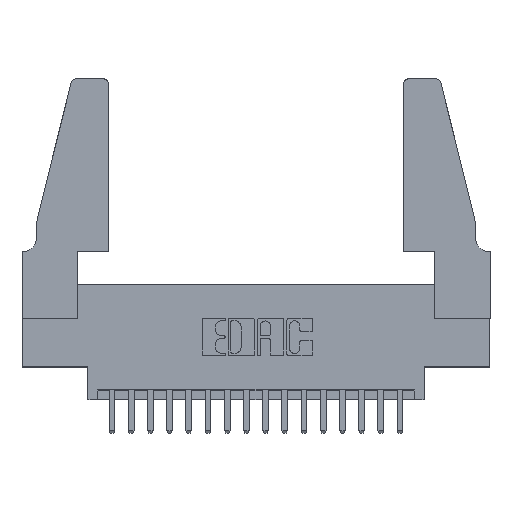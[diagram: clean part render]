
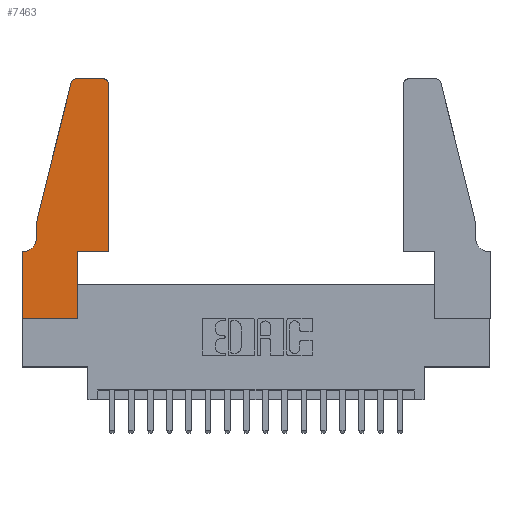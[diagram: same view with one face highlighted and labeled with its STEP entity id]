
A CAD part, top view. The second image highlights one B-rep face of the part: STEP entity #7463.
In plain terms, the highlighted planar face has unit normal (0, 0, 1).
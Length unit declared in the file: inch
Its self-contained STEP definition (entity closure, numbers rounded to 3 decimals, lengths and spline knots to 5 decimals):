
#109 = CARTESIAN_POINT ( 'NONE',  ( 0.0055, 0.35, 0.37 ) ) ;
#474 = ORIENTED_EDGE ( 'NONE', *, *, #11904, .T. ) ;
#642 = ORIENTED_EDGE ( 'NONE', *, *, #15482, .T. ) ;
#765 = DIRECTION ( 'NONE',  ( 0., 0., -1. ) ) ;
#843 = DIRECTION ( 'NONE',  ( -0.239, -0.971, 0. ) ) ;
#953 = LINE ( 'NONE', #1399, #3434 ) ;
#1150 = EDGE_CURVE ( 'NONE', #9525, #9662, #5143, .T. ) ;
#1267 = DIRECTION ( 'NONE',  ( 0., 1., 0. ) ) ;
#1284 = EDGE_CURVE ( 'NONE', #12994, #13766, #10468, .T. ) ;
#1294 = VECTOR ( 'NONE', #9110, 39.37008 ) ;
#1304 = CARTESIAN_POINT ( 'NONE',  ( 0.2605, 1.25, 0.37 ) ) ;
#1356 = ORIENTED_EDGE ( 'NONE', *, *, #17627, .T. ) ;
#1365 = LINE ( 'NONE', #4726, #8556 ) ;
#1399 = CARTESIAN_POINT ( 'NONE',  ( 0.4505, 0.35, 0.37 ) ) ;
#1490 = EDGE_CURVE ( 'NONE', #9662, #12390, #17792, .T. ) ;
#1530 = AXIS2_PLACEMENT_3D ( 'NONE', #3907, #13874, #5355 ) ;
#1618 = CARTESIAN_POINT ( 'NONE',  ( 0.0755, 0.5, 0.37 ) ) ;
#1721 = ORIENTED_EDGE ( 'NONE', *, *, #9318, .T. ) ;
#1859 = CARTESIAN_POINT ( 'NONE',  ( 0.2865, 0.35, 0.37 ) ) ;
#1992 = CARTESIAN_POINT ( 'NONE',  ( 0., 0., 0.37 ) ) ;
#2109 = DIRECTION ( 'NONE',  ( 1., 0., 0. ) ) ;
#2686 = CIRCLE ( 'NONE', #1530, 0.03 ) ;
#2865 = VECTOR ( 'NONE', #843, 39.37008 ) ;
#2963 = CARTESIAN_POINT ( 'NONE',  ( 0., 0.35, 0.37 ) ) ;
#3119 = AXIS2_PLACEMENT_3D ( 'NONE', #9359, #765, #10773 ) ;
#3434 = VECTOR ( 'NONE', #5691, 39.37008 ) ;
#3634 = EDGE_CURVE ( 'NONE', #13766, #15212, #13282, .T. ) ;
#3751 = LINE ( 'NONE', #10677, #18422 ) ;
#3825 = CARTESIAN_POINT ( 'NONE',  ( 0.2865, 0.35, 0.37 ) ) ;
#3907 = CARTESIAN_POINT ( 'NONE',  ( 0.284, 1.22, 0.37 ) ) ;
#3990 = LINE ( 'NONE', #1992, #6900 ) ;
#4007 = CARTESIAN_POINT ( 'NONE',  ( 0.0755, 0.42, 0.37 ) ) ;
#4099 = VERTEX_POINT ( 'NONE', #109 ) ;
#4253 = CARTESIAN_POINT ( 'NONE',  ( 0.4505, 1.22, 0.37 ) ) ;
#4267 = CARTESIAN_POINT ( 'NONE',  ( 0.284, 1.25, 0.37 ) ) ;
#4495 = DIRECTION ( 'NONE',  ( 1., 0., 0. ) ) ;
#4726 = CARTESIAN_POINT ( 'NONE',  ( 0.0755, 0.35, 0.37 ) ) ;
#5143 = LINE ( 'NONE', #15594, #1294 ) ;
#5355 = DIRECTION ( 'NONE',  ( 1., 0., 0. ) ) ;
#5691 = DIRECTION ( 'NONE',  ( 0., 1., 0. ) ) ;
#5715 = VECTOR ( 'NONE', #17340, 39.37008 ) ;
#5941 = CARTESIAN_POINT ( 'NONE',  ( 0.4205, 1.25, 0.37 ) ) ;
#5957 = EDGE_CURVE ( 'NONE', #12606, #12994, #2686, .T. ) ;
#6255 = DIRECTION ( 'NONE',  ( 0., 0., 1. ) ) ;
#6426 = EDGE_CURVE ( 'NONE', #12390, #6886, #3751, .T. ) ;
#6432 = CIRCLE ( 'NONE', #17276, 0.03 ) ;
#6886 = VERTEX_POINT ( 'NONE', #16083 ) ;
#6900 = VECTOR ( 'NONE', #14789, 39.37008 ) ;
#6916 = LINE ( 'NONE', #1304, #10248 ) ;
#7120 = EDGE_LOOP ( 'NONE', ( #474, #17174, #14389, #16852, #10218, #1721, #18307, #7163, #14049, #15892, #1356, #642 ) ) ;
#7163 = ORIENTED_EDGE ( 'NONE', *, *, #1150, .T. ) ;
#7463 = ADVANCED_FACE ( 'NONE', ( #16615 ), #10159, .T. ) ;
#8556 = VECTOR ( 'NONE', #9029, 39.37008 ) ;
#8744 = AXIS2_PLACEMENT_3D ( 'NONE', #2963, #13028, #4495 ) ;
#8820 = EDGE_CURVE ( 'NONE', #15212, #4099, #13684, .T. ) ;
#9029 = DIRECTION ( 'NONE',  ( -1., 0., 0. ) ) ;
#9110 = DIRECTION ( 'NONE',  ( 1., 0., 0. ) ) ;
#9318 = EDGE_CURVE ( 'NONE', #4099, #18301, #1365, .T. ) ;
#9359 = CARTESIAN_POINT ( 'NONE',  ( 0.0055, 0.42, 0.37 ) ) ;
#9525 = VERTEX_POINT ( 'NONE', #16526 ) ;
#9662 = VERTEX_POINT ( 'NONE', #15407 ) ;
#9889 = DIRECTION ( 'NONE',  ( -1., 0., 0. ) ) ;
#10159 = PLANE ( 'NONE',  #8744 ) ;
#10218 = ORIENTED_EDGE ( 'NONE', *, *, #8820, .T. ) ;
#10248 = VECTOR ( 'NONE', #9889, 39.37008 ) ;
#10468 = LINE ( 'NONE', #1618, #2865 ) ;
#10677 = CARTESIAN_POINT ( 'NONE',  ( 0.4505, 0.35, 0.37 ) ) ;
#10773 = DIRECTION ( 'NONE',  ( -1., 0., 0. ) ) ;
#11904 = EDGE_CURVE ( 'NONE', #12737, #12606, #6916, .T. ) ;
#12390 = VERTEX_POINT ( 'NONE', #3825 ) ;
#12606 = VERTEX_POINT ( 'NONE', #4267 ) ;
#12737 = VERTEX_POINT ( 'NONE', #5941 ) ;
#12952 = CARTESIAN_POINT ( 'NONE',  ( 0., 0.35, 0.37 ) ) ;
#12994 = VERTEX_POINT ( 'NONE', #16371 ) ;
#13028 = DIRECTION ( 'NONE',  ( 0., 0., 1. ) ) ;
#13139 = CARTESIAN_POINT ( 'NONE',  ( 0.0755, 0.5, 0.37 ) ) ;
#13282 = LINE ( 'NONE', #13139, #5715 ) ;
#13684 = CIRCLE ( 'NONE', #3119, 0.07 ) ;
#13766 = VERTEX_POINT ( 'NONE', #17023 ) ;
#13874 = DIRECTION ( 'NONE',  ( 0., 0., 1. ) ) ;
#14022 = VECTOR ( 'NONE', #1267, 39.37008 ) ;
#14049 = ORIENTED_EDGE ( 'NONE', *, *, #1490, .T. ) ;
#14389 = ORIENTED_EDGE ( 'NONE', *, *, #1284, .T. ) ;
#14778 = CARTESIAN_POINT ( 'NONE',  ( 0.4205, 1.22, 0.37 ) ) ;
#14789 = DIRECTION ( 'NONE',  ( 0., -1., 0. ) ) ;
#14945 = EDGE_CURVE ( 'NONE', #18301, #9525, #3990, .T. ) ;
#15212 = VERTEX_POINT ( 'NONE', #4007 ) ;
#15407 = CARTESIAN_POINT ( 'NONE',  ( 0.2865, 0., 0.37 ) ) ;
#15482 = EDGE_CURVE ( 'NONE', #15909, #12737, #6432, .T. ) ;
#15594 = CARTESIAN_POINT ( 'NONE',  ( 0., 0., 0.37 ) ) ;
#15892 = ORIENTED_EDGE ( 'NONE', *, *, #6426, .T. ) ;
#15909 = VERTEX_POINT ( 'NONE', #4253 ) ;
#16083 = CARTESIAN_POINT ( 'NONE',  ( 0.4505, 0.35, 0.37 ) ) ;
#16199 = DIRECTION ( 'NONE',  ( 1., 0., 0. ) ) ;
#16371 = CARTESIAN_POINT ( 'NONE',  ( 0.25487, 1.22718, 0.37 ) ) ;
#16526 = CARTESIAN_POINT ( 'NONE',  ( 0., 0., 0.37 ) ) ;
#16615 = FACE_OUTER_BOUND ( 'NONE', #7120, .T. ) ;
#16852 = ORIENTED_EDGE ( 'NONE', *, *, #3634, .T. ) ;
#17023 = CARTESIAN_POINT ( 'NONE',  ( 0.0755, 0.5, 0.37 ) ) ;
#17174 = ORIENTED_EDGE ( 'NONE', *, *, #5957, .T. ) ;
#17276 = AXIS2_PLACEMENT_3D ( 'NONE', #14778, #6255, #16199 ) ;
#17340 = DIRECTION ( 'NONE',  ( 0., -1., 0. ) ) ;
#17627 = EDGE_CURVE ( 'NONE', #6886, #15909, #953, .T. ) ;
#17792 = LINE ( 'NONE', #1859, #14022 ) ;
#18301 = VERTEX_POINT ( 'NONE', #12952 ) ;
#18307 = ORIENTED_EDGE ( 'NONE', *, *, #14945, .T. ) ;
#18422 = VECTOR ( 'NONE', #2109, 39.37008 ) ;
